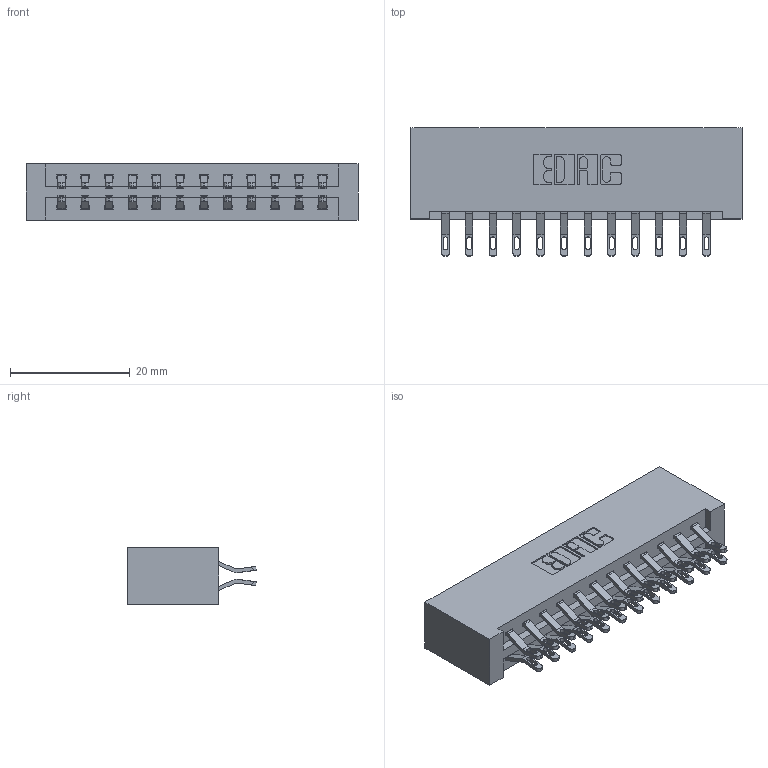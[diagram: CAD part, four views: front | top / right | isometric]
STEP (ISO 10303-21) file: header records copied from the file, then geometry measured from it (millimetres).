
FILE_DESCRIPTION (( 'STEP AP203' ), '1' );
FILE_NAME ('337-024-555-201.STEP', '2018-08-06T01:32:37', ( '' ), ( '' ), 'SwSTEP 2.0', 'SolidWorks 2016', '' );
FILE_SCHEMA (( 'CONFIG_CONTROL_DESIGN' ));
Length unit declared in the file: inch
Products named in the file (3): 337 Part_No Mounting Lugs; 345-292-001_555 Tail; 337-024-555-201
Assembly tree (25 placements, depth 2):
  337-024-555-201
    337 Part_No Mounting Lugs
    345-292-001_555 Tail  x24
Bounding box: 55.42 x 21.47 x 9.4 mm (x, y, z)
Volume: 6271.9 mm3; surface area: 7117.4 mm2
Topology: 25 solids, 25 shells, 1546 faces, 4823 edges, 3214 vertices
Faces by surface type: plane 930, cylinder 616
Entity records: 13233 total; most frequent: CARTESIAN_POINT 2288, ORIENTED_EDGE 2194, DIRECTION 1965, EDGE_CURVE 1097, VECTOR 957, LINE 957, VERTEX_POINT 730, AXIS2_PLACEMENT_3D 504
